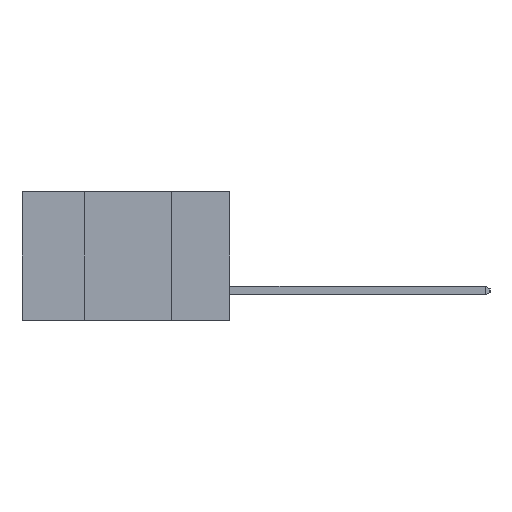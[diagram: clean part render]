
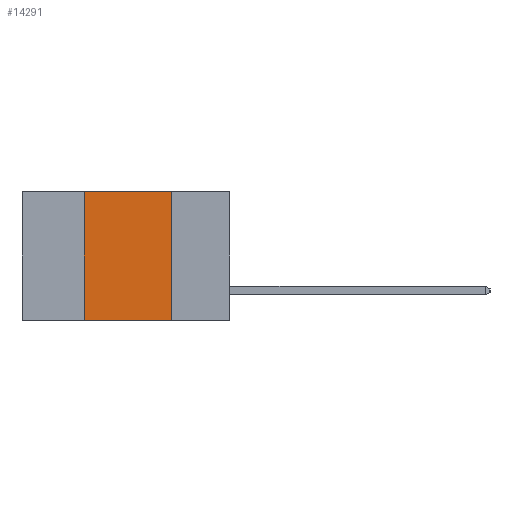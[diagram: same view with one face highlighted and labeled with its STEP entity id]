
A CAD part, left-side view. The second image highlights one B-rep face of the part: STEP entity #14291.
In plain terms, the highlighted planar face has unit normal (-1, 0, 0).
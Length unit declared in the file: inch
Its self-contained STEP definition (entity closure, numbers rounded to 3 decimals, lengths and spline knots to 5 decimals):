
#460 = CARTESIAN_POINT ( 'NONE',  ( 0., 0.17, 0. ) ) ;
#803 = CARTESIAN_POINT ( 'NONE',  ( 0., 0.6, 0. ) ) ;
#1721 = ORIENTED_EDGE ( 'NONE', *, *, #9267, .T. ) ;
#2260 = VERTEX_POINT ( 'NONE', #7746 ) ;
#2290 = DIRECTION ( 'NONE',  ( 0., 0., -1. ) ) ;
#3575 = ORIENTED_EDGE ( 'NONE', *, *, #17350, .F. ) ;
#3629 = ORIENTED_EDGE ( 'NONE', *, *, #14555, .F. ) ;
#4297 = DIRECTION ( 'NONE',  ( 0., -1., 0. ) ) ;
#5673 = AXIS2_PLACEMENT_3D ( 'NONE', #803, #10984, #2290 ) ;
#5918 = LINE ( 'NONE', #17262, #17303 ) ;
#6665 = PLANE ( 'NONE',  #5673 ) ;
#6751 = VERTEX_POINT ( 'NONE', #10862 ) ;
#6837 = EDGE_CURVE ( 'NONE', #16600, #2260, #18234, .T. ) ;
#6902 = VECTOR ( 'NONE', #9603, 39.37008 ) ;
#7414 = VECTOR ( 'NONE', #12296, 39.37008 ) ;
#7746 = CARTESIAN_POINT ( 'NONE',  ( 0., 0.17, -0.37 ) ) ;
#7939 = CARTESIAN_POINT ( 'NONE',  ( 0., 0.6, 0. ) ) ;
#8733 = DIRECTION ( 'NONE',  ( 0., 0., 1. ) ) ;
#9267 = EDGE_CURVE ( 'NONE', #6751, #2260, #16071, .T. ) ;
#9603 = DIRECTION ( 'NONE',  ( 0., 0., -1. ) ) ;
#10027 = CARTESIAN_POINT ( 'NONE',  ( 0., 0.6, -0.37 ) ) ;
#10236 = CARTESIAN_POINT ( 'NONE',  ( 0., 0.17, -0.37 ) ) ;
#10862 = CARTESIAN_POINT ( 'NONE',  ( 0., 0.42, -0.37 ) ) ;
#10984 = DIRECTION ( 'NONE',  ( 1., 0., 0. ) ) ;
#12257 = VECTOR ( 'NONE', #4297, 39.37008 ) ;
#12296 = DIRECTION ( 'NONE',  ( 0., -1., 0. ) ) ;
#12851 = ORIENTED_EDGE ( 'NONE', *, *, #6837, .F. ) ;
#14247 = FACE_OUTER_BOUND ( 'NONE', #15558, .T. ) ;
#14291 = ADVANCED_FACE ( 'NONE', ( #14247 ), #6665, .F. ) ;
#14555 = EDGE_CURVE ( 'NONE', #6751, #18238, #5918, .T. ) ;
#15516 = LINE ( 'NONE', #7939, #7414 ) ;
#15558 = EDGE_LOOP ( 'NONE', ( #12851, #3575, #3629, #1721 ) ) ;
#15968 = CARTESIAN_POINT ( 'NONE',  ( 0., 0.42, 0. ) ) ;
#16071 = LINE ( 'NONE', #10027, #12257 ) ;
#16600 = VERTEX_POINT ( 'NONE', #460 ) ;
#17262 = CARTESIAN_POINT ( 'NONE',  ( 0., 0.42, -0.37 ) ) ;
#17303 = VECTOR ( 'NONE', #8733, 39.37008 ) ;
#17350 = EDGE_CURVE ( 'NONE', #18238, #16600, #15516, .T. ) ;
#18234 = LINE ( 'NONE', #10236, #6902 ) ;
#18238 = VERTEX_POINT ( 'NONE', #15968 ) ;
